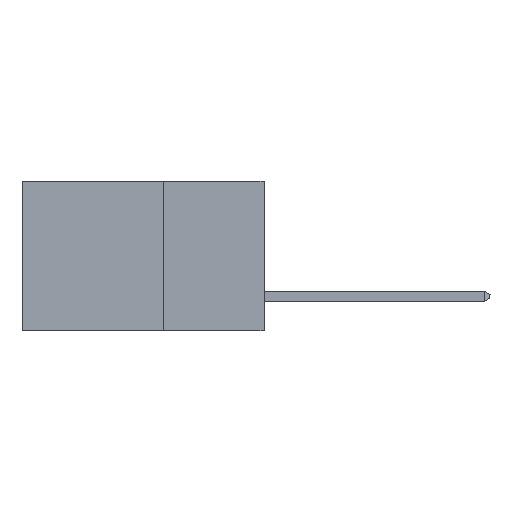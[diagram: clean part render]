
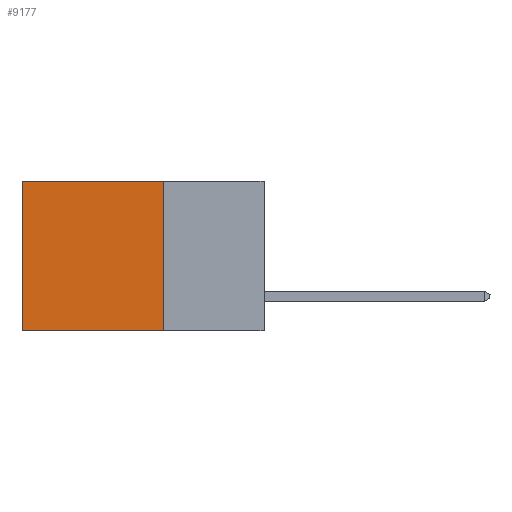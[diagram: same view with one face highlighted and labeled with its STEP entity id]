
A CAD part, left-side view. The second image highlights one B-rep face of the part: STEP entity #9177.
In plain terms, the highlighted planar face has unit normal (-1, 0, 0).
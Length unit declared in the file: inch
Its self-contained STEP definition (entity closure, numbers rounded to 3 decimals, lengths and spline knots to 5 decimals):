
#386 = VERTEX_POINT ( 'NONE', #7267 ) ;
#442 = CARTESIAN_POINT ( 'NONE',  ( 0.2615, 0.25, 0. ) ) ;
#542 = CARTESIAN_POINT ( 'NONE',  ( 0.2615, 0.25, -0.37 ) ) ;
#981 = VECTOR ( 'NONE', #1999, 39.37008 ) ;
#1508 = CARTESIAN_POINT ( 'NONE',  ( 0.2615, 0.6, -0.37 ) ) ;
#1719 = CARTESIAN_POINT ( 'NONE',  ( 0.2615, 0.25, 0. ) ) ;
#1999 = DIRECTION ( 'NONE',  ( 0., 0., -1. ) ) ;
#2299 = ORIENTED_EDGE ( 'NONE', *, *, #6077, .F. ) ;
#3373 = DIRECTION ( 'NONE',  ( 0., 0., -1. ) ) ;
#3878 = LINE ( 'NONE', #1719, #5321 ) ;
#4006 = AXIS2_PLACEMENT_3D ( 'NONE', #4307, #11612, #3373 ) ;
#4016 = VECTOR ( 'NONE', #11728, 39.37008 ) ;
#4307 = CARTESIAN_POINT ( 'NONE',  ( 0.2615, 0.25, -0.37 ) ) ;
#4569 = LINE ( 'NONE', #542, #5672 ) ;
#5009 = CARTESIAN_POINT ( 'NONE',  ( 0.2615, 0.6, -0.37 ) ) ;
#5211 = ORIENTED_EDGE ( 'NONE', *, *, #9429, .T. ) ;
#5321 = VECTOR ( 'NONE', #11735, 39.37008 ) ;
#5672 = VECTOR ( 'NONE', #8570, 39.37008 ) ;
#6077 = EDGE_CURVE ( 'NONE', #6467, #11238, #4569, .T. ) ;
#6356 = VERTEX_POINT ( 'NONE', #1508 ) ;
#6467 = VERTEX_POINT ( 'NONE', #442 ) ;
#6560 = PLANE ( 'NONE',  #4006 ) ;
#7095 = LINE ( 'NONE', #5009, #981 ) ;
#7267 = CARTESIAN_POINT ( 'NONE',  ( 0.2615, 0.6, 0. ) ) ;
#7732 = LINE ( 'NONE', #10908, #4016 ) ;
#7994 = CARTESIAN_POINT ( 'NONE',  ( 0.2615, 0.25, -0.37 ) ) ;
#8570 = DIRECTION ( 'NONE',  ( 0., 0., -1. ) ) ;
#9177 = ADVANCED_FACE ( 'NONE', ( #10469 ), #6560, .F. ) ;
#9429 = EDGE_CURVE ( 'NONE', #386, #6356, #7095, .T. ) ;
#9700 = EDGE_CURVE ( 'NONE', #11238, #6356, #7732, .T. ) ;
#9765 = ORIENTED_EDGE ( 'NONE', *, *, #9700, .F. ) ;
#10469 = FACE_OUTER_BOUND ( 'NONE', #12231, .T. ) ;
#10482 = ORIENTED_EDGE ( 'NONE', *, *, #12345, .T. ) ;
#10908 = CARTESIAN_POINT ( 'NONE',  ( 0.2615, 0.25, -0.37 ) ) ;
#11238 = VERTEX_POINT ( 'NONE', #7994 ) ;
#11612 = DIRECTION ( 'NONE',  ( 1., 0., 0. ) ) ;
#11728 = DIRECTION ( 'NONE',  ( 0., 1., 0. ) ) ;
#11735 = DIRECTION ( 'NONE',  ( 0., 1., 0. ) ) ;
#12231 = EDGE_LOOP ( 'NONE', ( #5211, #9765, #2299, #10482 ) ) ;
#12345 = EDGE_CURVE ( 'NONE', #6467, #386, #3878, .T. ) ;
